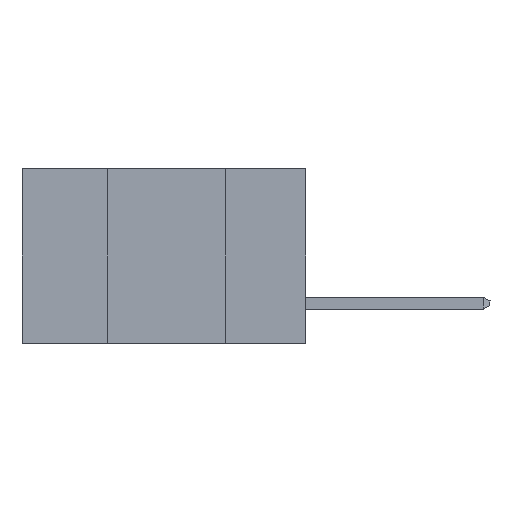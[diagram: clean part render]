
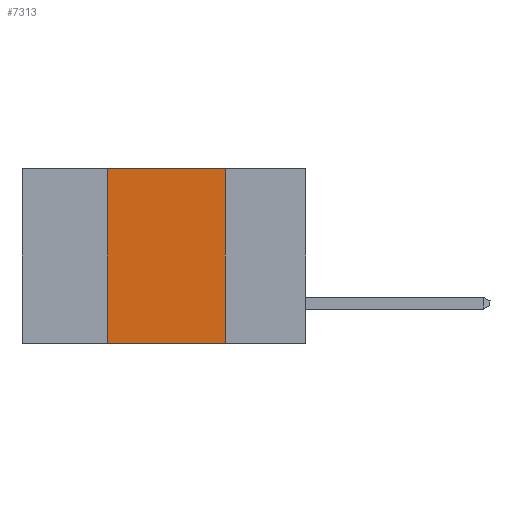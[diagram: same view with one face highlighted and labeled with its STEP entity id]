
A CAD part, left-side view. The second image highlights one B-rep face of the part: STEP entity #7313.
In plain terms, the highlighted planar face has unit normal (-1, 0, 0).
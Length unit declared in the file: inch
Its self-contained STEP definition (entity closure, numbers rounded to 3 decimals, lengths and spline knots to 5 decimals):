
#3132 = EDGE_CURVE ( 'NONE', #5881, #12178, #20554, .T. ) ;
#3232 = FACE_OUTER_BOUND ( 'NONE', #8916, .T. ) ;
#3236 = CARTESIAN_POINT ( 'NONE',  ( 0., 0.17, 0. ) ) ;
#3550 = LINE ( 'NONE', #16509, #20259 ) ;
#5782 = LINE ( 'NONE', #25503, #7557 ) ;
#5881 = VERTEX_POINT ( 'NONE', #26854 ) ;
#6448 = EDGE_CURVE ( 'NONE', #17202, #12178, #22463, .T. ) ;
#6781 = CARTESIAN_POINT ( 'NONE',  ( 0., 0.6, 0. ) ) ;
#7313 = ADVANCED_FACE ( 'NONE', ( #3232 ), #18092, .F. ) ;
#7557 = VECTOR ( 'NONE', #20813, 39.37008 ) ;
#8588 = CARTESIAN_POINT ( 'NONE',  ( 0., 0.6, -0.37 ) ) ;
#8916 = EDGE_LOOP ( 'NONE', ( #27264, #17646, #18273, #16617 ) ) ;
#12178 = VERTEX_POINT ( 'NONE', #29161 ) ;
#13038 = DIRECTION ( 'NONE',  ( 0., -1., 0. ) ) ;
#13195 = CARTESIAN_POINT ( 'NONE',  ( 0., 0.17, 0. ) ) ;
#13523 = CARTESIAN_POINT ( 'NONE',  ( 0., 0.42, 0. ) ) ;
#15509 = DIRECTION ( 'NONE',  ( 0., 0., -1. ) ) ;
#16509 = CARTESIAN_POINT ( 'NONE',  ( 0., 0.42, 0. ) ) ;
#16617 = ORIENTED_EDGE ( 'NONE', *, *, #3132, .T. ) ;
#17202 = VERTEX_POINT ( 'NONE', #3236 ) ;
#17646 = ORIENTED_EDGE ( 'NONE', *, *, #25582, .F. ) ;
#17716 = EDGE_CURVE ( 'NONE', #5881, #23640, #3550, .T. ) ;
#18057 = VECTOR ( 'NONE', #13038, 39.37008 ) ;
#18092 = PLANE ( 'NONE',  #25366 ) ;
#18273 = ORIENTED_EDGE ( 'NONE', *, *, #17716, .F. ) ;
#20259 = VECTOR ( 'NONE', #25852, 39.37008 ) ;
#20554 = LINE ( 'NONE', #8588, #18057 ) ;
#20813 = DIRECTION ( 'NONE',  ( 0., -1., 0. ) ) ;
#22463 = LINE ( 'NONE', #13195, #25665 ) ;
#22690 = DIRECTION ( 'NONE',  ( 1., 0., 0. ) ) ;
#23640 = VERTEX_POINT ( 'NONE', #13523 ) ;
#25366 = AXIS2_PLACEMENT_3D ( 'NONE', #6781, #22690, #27120 ) ;
#25503 = CARTESIAN_POINT ( 'NONE',  ( 0., 0.6, 0. ) ) ;
#25582 = EDGE_CURVE ( 'NONE', #23640, #17202, #5782, .T. ) ;
#25665 = VECTOR ( 'NONE', #15509, 39.37008 ) ;
#25852 = DIRECTION ( 'NONE',  ( 0., 0., 1. ) ) ;
#26854 = CARTESIAN_POINT ( 'NONE',  ( 0., 0.42, -0.37 ) ) ;
#27120 = DIRECTION ( 'NONE',  ( 0., 0., -1. ) ) ;
#27264 = ORIENTED_EDGE ( 'NONE', *, *, #6448, .F. ) ;
#29161 = CARTESIAN_POINT ( 'NONE',  ( 0., 0.17, -0.37 ) ) ;
